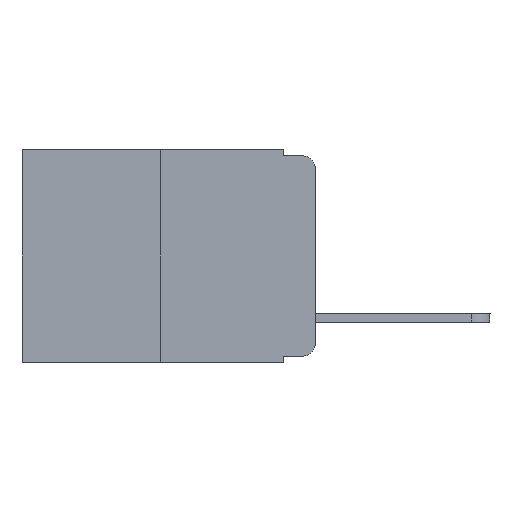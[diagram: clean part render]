
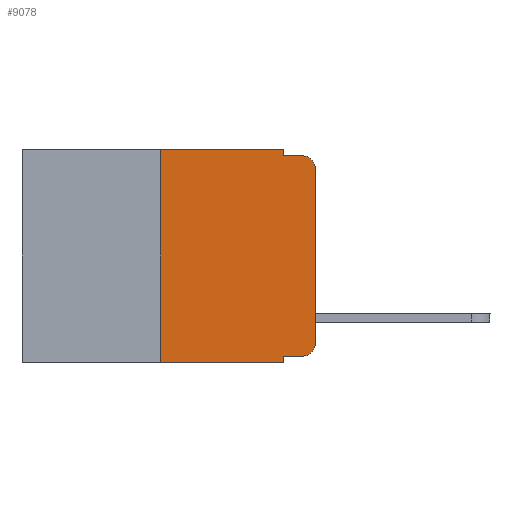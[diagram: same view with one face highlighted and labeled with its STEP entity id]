
A CAD part, left-side view. The second image highlights one B-rep face of the part: STEP entity #9078.
In plain terms, the highlighted planar face has unit normal (-1, 0, 0).
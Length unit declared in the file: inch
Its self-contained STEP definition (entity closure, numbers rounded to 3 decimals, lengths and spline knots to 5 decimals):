
#144 = EDGE_CURVE ( 'NONE', #7556, #10414, #6288, .T. ) ;
#226 = VECTOR ( 'NONE', #604, 39.37008 ) ;
#342 = LINE ( 'NONE', #6030, #3443 ) ;
#356 = CARTESIAN_POINT ( 'NONE',  ( 0., 0.051, -0.01 ) ) ;
#481 = AXIS2_PLACEMENT_3D ( 'NONE', #9605, #15279, #12408 ) ;
#573 = EDGE_CURVE ( 'NONE', #13741, #10414, #8477, .T. ) ;
#604 = DIRECTION ( 'NONE',  ( 0., -1., 0. ) ) ;
#645 = ORIENTED_EDGE ( 'NONE', *, *, #18365, .T. ) ;
#1344 = EDGE_CURVE ( 'NONE', #15001, #16042, #16729, .T. ) ;
#1438 = CARTESIAN_POINT ( 'NONE',  ( 0., 0., -0.313 ) ) ;
#1515 = DIRECTION ( 'NONE',  ( -1., 0., 0. ) ) ;
#1547 = VERTEX_POINT ( 'NONE', #17397 ) ;
#1825 = CARTESIAN_POINT ( 'NONE',  ( 0., 0.051, 0. ) ) ;
#1911 = DIRECTION ( 'NONE',  ( 0., -1., 0. ) ) ;
#1923 = ORIENTED_EDGE ( 'NONE', *, *, #3212, .F. ) ;
#2279 = EDGE_CURVE ( 'NONE', #16042, #7556, #10673, .T. ) ;
#2320 = VECTOR ( 'NONE', #8268, 39.37008 ) ;
#2456 = PLANE ( 'NONE',  #481 ) ;
#2811 = EDGE_LOOP ( 'NONE', ( #17225, #10705, #17922, #8051, #10833, #6937, #12259, #1923, #645, #2961 ) ) ;
#2835 = DIRECTION ( 'NONE',  ( 0., 0., 1. ) ) ;
#2961 = ORIENTED_EDGE ( 'NONE', *, *, #1344, .T. ) ;
#3032 = VERTEX_POINT ( 'NONE', #16283 ) ;
#3065 = CARTESIAN_POINT ( 'NONE',  ( 0., 0.051, -0.01 ) ) ;
#3156 = VECTOR ( 'NONE', #8019, 39.37008 ) ;
#3195 = CARTESIAN_POINT ( 'NONE',  ( 0., 0.25, 0. ) ) ;
#3212 = EDGE_CURVE ( 'NONE', #1547, #8909, #7041, .T. ) ;
#3304 = VECTOR ( 'NONE', #2835, 39.37008 ) ;
#3443 = VECTOR ( 'NONE', #1911, 39.37008 ) ;
#3781 = EDGE_CURVE ( 'NONE', #3032, #14730, #17291, .T. ) ;
#4203 = LINE ( 'NONE', #13311, #226 ) ;
#4434 = AXIS2_PLACEMENT_3D ( 'NONE', #17152, #1515, #12990 ) ;
#4726 = LINE ( 'NONE', #5752, #2320 ) ;
#4839 = CARTESIAN_POINT ( 'NONE',  ( 0., 0.25, 0. ) ) ;
#5231 = AXIS2_PLACEMENT_3D ( 'NONE', #10111, #10298, #17276 ) ;
#5735 = VECTOR ( 'NONE', #8983, 39.37008 ) ;
#5752 = CARTESIAN_POINT ( 'NONE',  ( 0., 0.051, 0. ) ) ;
#6030 = CARTESIAN_POINT ( 'NONE',  ( 0., 0.473, 0. ) ) ;
#6288 = CIRCLE ( 'NONE', #5231, 0.02 ) ;
#6586 = CARTESIAN_POINT ( 'NONE',  ( 0., 0., 0. ) ) ;
#6937 = ORIENTED_EDGE ( 'NONE', *, *, #3781, .F. ) ;
#7041 = LINE ( 'NONE', #1825, #5735 ) ;
#7401 = EDGE_CURVE ( 'NONE', #15227, #13741, #4726, .T. ) ;
#7556 = VERTEX_POINT ( 'NONE', #17325 ) ;
#8019 = DIRECTION ( 'NONE',  ( 0., 0., 1. ) ) ;
#8049 = VECTOR ( 'NONE', #15862, 39.37008 ) ;
#8051 = ORIENTED_EDGE ( 'NONE', *, *, #7401, .F. ) ;
#8268 = DIRECTION ( 'NONE',  ( 0., 0., -1. ) ) ;
#8477 = LINE ( 'NONE', #356, #8049 ) ;
#8909 = VERTEX_POINT ( 'NONE', #12040 ) ;
#8983 = DIRECTION ( 'NONE',  ( 0., 0., -1. ) ) ;
#9078 = ADVANCED_FACE ( 'NONE', ( #12780 ), #2456, .F. ) ;
#9140 = VECTOR ( 'NONE', #15876, 39.37008 ) ;
#9605 = CARTESIAN_POINT ( 'NONE',  ( 0., 0.473, 0. ) ) ;
#9781 = CARTESIAN_POINT ( 'NONE',  ( 0., 0.02, -0.01 ) ) ;
#9810 = LINE ( 'NONE', #11402, #9140 ) ;
#10111 = CARTESIAN_POINT ( 'NONE',  ( 0., 0.02, -0.03 ) ) ;
#10298 = DIRECTION ( 'NONE',  ( -1., 0., 0. ) ) ;
#10414 = VERTEX_POINT ( 'NONE', #9781 ) ;
#10673 = LINE ( 'NONE', #6586, #3156 ) ;
#10705 = ORIENTED_EDGE ( 'NONE', *, *, #144, .T. ) ;
#10833 = ORIENTED_EDGE ( 'NONE', *, *, #17420, .F. ) ;
#11402 = CARTESIAN_POINT ( 'NONE',  ( 0., 0.051, -0.333 ) ) ;
#12040 = CARTESIAN_POINT ( 'NONE',  ( 0., 0.051, -0.343 ) ) ;
#12259 = ORIENTED_EDGE ( 'NONE', *, *, #14218, .T. ) ;
#12408 = DIRECTION ( 'NONE',  ( 0., 0., -1. ) ) ;
#12780 = FACE_OUTER_BOUND ( 'NONE', #2811, .T. ) ;
#12990 = DIRECTION ( 'NONE',  ( 0., 0., -1. ) ) ;
#13311 = CARTESIAN_POINT ( 'NONE',  ( 0., 0.473, -0.343 ) ) ;
#13716 = CARTESIAN_POINT ( 'NONE',  ( 0., 0.02, -0.333 ) ) ;
#13741 = VERTEX_POINT ( 'NONE', #3065 ) ;
#14218 = EDGE_CURVE ( 'NONE', #3032, #8909, #4203, .T. ) ;
#14730 = VERTEX_POINT ( 'NONE', #3195 ) ;
#15001 = VERTEX_POINT ( 'NONE', #13716 ) ;
#15227 = VERTEX_POINT ( 'NONE', #16624 ) ;
#15279 = DIRECTION ( 'NONE',  ( 1., 0., 0. ) ) ;
#15862 = DIRECTION ( 'NONE',  ( 0., -1., 0. ) ) ;
#15876 = DIRECTION ( 'NONE',  ( 0., -1., 0. ) ) ;
#16042 = VERTEX_POINT ( 'NONE', #1438 ) ;
#16283 = CARTESIAN_POINT ( 'NONE',  ( 0., 0.25, -0.343 ) ) ;
#16624 = CARTESIAN_POINT ( 'NONE',  ( 0., 0.051, 0. ) ) ;
#16729 = CIRCLE ( 'NONE', #4434, 0.02 ) ;
#17152 = CARTESIAN_POINT ( 'NONE',  ( 0., 0.02, -0.313 ) ) ;
#17225 = ORIENTED_EDGE ( 'NONE', *, *, #2279, .T. ) ;
#17276 = DIRECTION ( 'NONE',  ( 0., 0., -1. ) ) ;
#17291 = LINE ( 'NONE', #4839, #3304 ) ;
#17325 = CARTESIAN_POINT ( 'NONE',  ( 0., 0., -0.03 ) ) ;
#17397 = CARTESIAN_POINT ( 'NONE',  ( 0., 0.051, -0.333 ) ) ;
#17420 = EDGE_CURVE ( 'NONE', #14730, #15227, #342, .T. ) ;
#17922 = ORIENTED_EDGE ( 'NONE', *, *, #573, .F. ) ;
#18365 = EDGE_CURVE ( 'NONE', #1547, #15001, #9810, .T. ) ;
